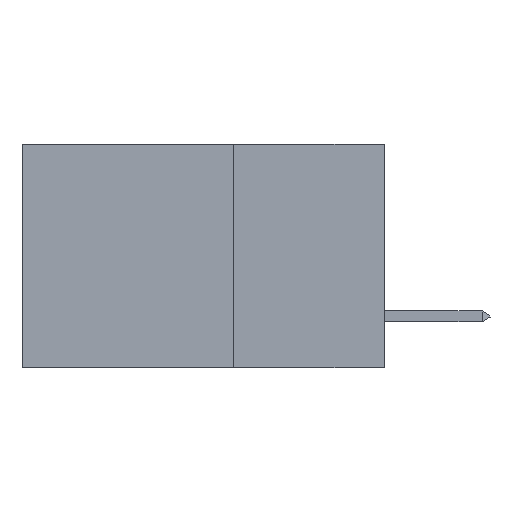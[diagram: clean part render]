
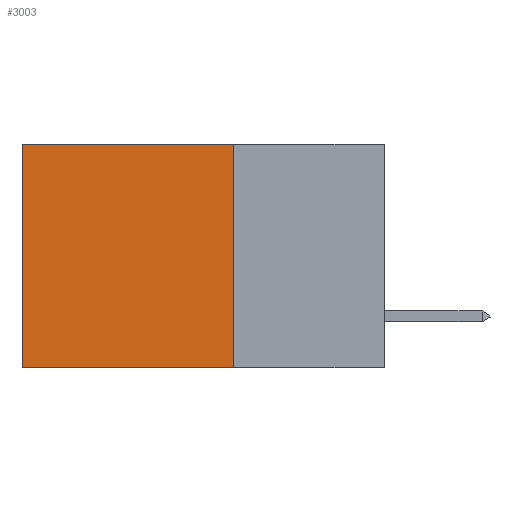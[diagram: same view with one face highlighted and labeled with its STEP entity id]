
A CAD part, left-side view. The second image highlights one B-rep face of the part: STEP entity #3003.
In plain terms, the highlighted planar face has unit normal (-1, 0, 0).
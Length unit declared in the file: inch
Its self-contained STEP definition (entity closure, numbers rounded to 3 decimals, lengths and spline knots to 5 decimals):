
#61 = CARTESIAN_POINT ( 'NONE',  ( 0.2875, 0.6, -0.37 ) ) ;
#197 = VECTOR ( 'NONE', #1210, 39.37008 ) ;
#787 = VERTEX_POINT ( 'NONE', #13059 ) ;
#800 = VERTEX_POINT ( 'NONE', #61 ) ;
#1202 = DIRECTION ( 'NONE',  ( 1., 0., 0. ) ) ;
#1210 = DIRECTION ( 'NONE',  ( 0., 1., 0. ) ) ;
#1248 = LINE ( 'NONE', #3622, #11842 ) ;
#1331 = DIRECTION ( 'NONE',  ( 0., 0., -1. ) ) ;
#1392 = CARTESIAN_POINT ( 'NONE',  ( 0.2875, 0.25, 0. ) ) ;
#1927 = ORIENTED_EDGE ( 'NONE', *, *, #15795, .T. ) ;
#2277 = VERTEX_POINT ( 'NONE', #7526 ) ;
#2408 = VECTOR ( 'NONE', #10609, 39.37008 ) ;
#2846 = LINE ( 'NONE', #10547, #2408 ) ;
#3003 = ADVANCED_FACE ( 'NONE', ( #16734 ), #17218, .F. ) ;
#3622 = CARTESIAN_POINT ( 'NONE',  ( 0.2875, 0.6, 0. ) ) ;
#4224 = EDGE_CURVE ( 'NONE', #2277, #17962, #16676, .T. ) ;
#5127 = DIRECTION ( 'NONE',  ( 0., 1., 0. ) ) ;
#5507 = CARTESIAN_POINT ( 'NONE',  ( 0.2875, 0.25, 0. ) ) ;
#5831 = EDGE_CURVE ( 'NONE', #787, #800, #6123, .T. ) ;
#6123 = LINE ( 'NONE', #10972, #14720 ) ;
#6294 = ORIENTED_EDGE ( 'NONE', *, *, #5831, .F. ) ;
#7454 = AXIS2_PLACEMENT_3D ( 'NONE', #1392, #1202, #1331 ) ;
#7478 = ORIENTED_EDGE ( 'NONE', *, *, #10072, .F. ) ;
#7526 = CARTESIAN_POINT ( 'NONE',  ( 0.2875, 0.25, 0. ) ) ;
#10072 = EDGE_CURVE ( 'NONE', #2277, #787, #2846, .T. ) ;
#10377 = ORIENTED_EDGE ( 'NONE', *, *, #4224, .T. ) ;
#10547 = CARTESIAN_POINT ( 'NONE',  ( 0.2875, 0.25, 0. ) ) ;
#10609 = DIRECTION ( 'NONE',  ( 0., 0., -1. ) ) ;
#10972 = CARTESIAN_POINT ( 'NONE',  ( 0.2875, 0.25, -0.37 ) ) ;
#11842 = VECTOR ( 'NONE', #16519, 39.37008 ) ;
#13059 = CARTESIAN_POINT ( 'NONE',  ( 0.2875, 0.25, -0.37 ) ) ;
#13449 = EDGE_LOOP ( 'NONE', ( #1927, #6294, #7478, #10377 ) ) ;
#14720 = VECTOR ( 'NONE', #5127, 39.37008 ) ;
#15795 = EDGE_CURVE ( 'NONE', #17962, #800, #1248, .T. ) ;
#16519 = DIRECTION ( 'NONE',  ( 0., 0., -1. ) ) ;
#16676 = LINE ( 'NONE', #5507, #197 ) ;
#16734 = FACE_OUTER_BOUND ( 'NONE', #13449, .T. ) ;
#16974 = CARTESIAN_POINT ( 'NONE',  ( 0.2875, 0.6, 0. ) ) ;
#17218 = PLANE ( 'NONE',  #7454 ) ;
#17962 = VERTEX_POINT ( 'NONE', #16974 ) ;
